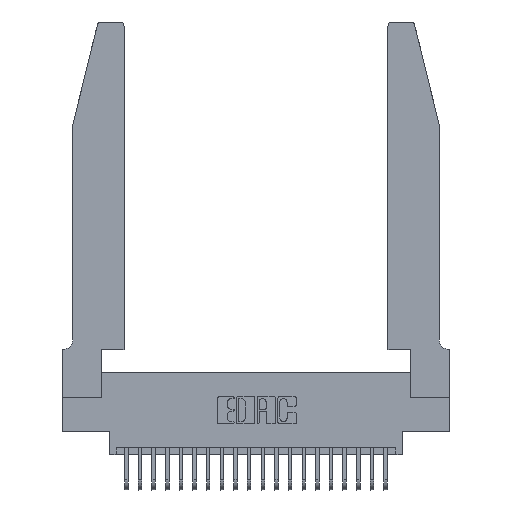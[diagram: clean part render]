
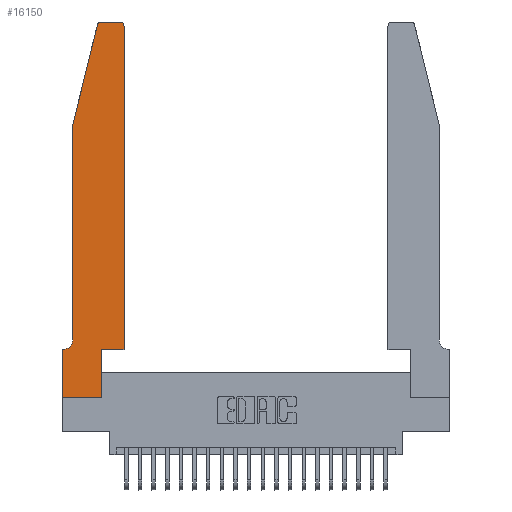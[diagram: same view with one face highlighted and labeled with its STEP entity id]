
A CAD part, top view. The second image highlights one B-rep face of the part: STEP entity #16150.
In plain terms, the highlighted planar face has unit normal (0, 0, 1).
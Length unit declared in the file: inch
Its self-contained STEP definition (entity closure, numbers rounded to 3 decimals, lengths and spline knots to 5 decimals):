
#23 = CARTESIAN_POINT ( 'NONE',  ( 0.25487, 2.72718, 0.37 ) ) ;
#61 = VERTEX_POINT ( 'NONE', #21375 ) ;
#76 = EDGE_CURVE ( 'NONE', #13377, #61, #11208, .T. ) ;
#625 = EDGE_LOOP ( 'NONE', ( #3779, #20470, #11960, #14670, #16155, #15663, #4554, #1819, #11596, #8665, #4752, #5791 ) ) ;
#868 = DIRECTION ( 'NONE',  ( -0.239, -0.971, 0. ) ) ;
#911 = EDGE_CURVE ( 'NONE', #7710, #11532, #14795, .T. ) ;
#967 = LINE ( 'NONE', #7769, #9959 ) ;
#1411 = DIRECTION ( 'NONE',  ( -1., 0., 0. ) ) ;
#1785 = VERTEX_POINT ( 'NONE', #6519 ) ;
#1819 = ORIENTED_EDGE ( 'NONE', *, *, #5611, .T. ) ;
#1923 = CARTESIAN_POINT ( 'NONE',  ( 0.2865, 0.35, 0.37 ) ) ;
#2019 = DIRECTION ( 'NONE',  ( 0., 0., 1. ) ) ;
#3181 = CARTESIAN_POINT ( 'NONE',  ( 0.2865, 0., 0.37 ) ) ;
#3467 = VECTOR ( 'NONE', #868, 39.37008 ) ;
#3557 = LINE ( 'NONE', #11587, #8333 ) ;
#3666 = DIRECTION ( 'NONE',  ( 0., 1., 0. ) ) ;
#3731 = CARTESIAN_POINT ( 'NONE',  ( 0., 0.35, 0.37 ) ) ;
#3779 = ORIENTED_EDGE ( 'NONE', *, *, #5363, .T. ) ;
#3974 = VERTEX_POINT ( 'NONE', #16724 ) ;
#4528 = EDGE_CURVE ( 'NONE', #19229, #3974, #967, .T. ) ;
#4554 = ORIENTED_EDGE ( 'NONE', *, *, #14493, .T. ) ;
#4644 = EDGE_CURVE ( 'NONE', #18680, #19229, #3557, .T. ) ;
#4752 = ORIENTED_EDGE ( 'NONE', *, *, #4528, .T. ) ;
#4996 = EDGE_CURVE ( 'NONE', #8780, #18680, #18169, .T. ) ;
#5137 = VERTEX_POINT ( 'NONE', #11493 ) ;
#5363 = EDGE_CURVE ( 'NONE', #1785, #21702, #6318, .T. ) ;
#5474 = CARTESIAN_POINT ( 'NONE',  ( 0.4505, 0.35, 0.37 ) ) ;
#5552 = DIRECTION ( 'NONE',  ( 1., 0., 0. ) ) ;
#5611 = EDGE_CURVE ( 'NONE', #5137, #8780, #15953, .T. ) ;
#5791 = ORIENTED_EDGE ( 'NONE', *, *, #6215, .T. ) ;
#6003 = AXIS2_PLACEMENT_3D ( 'NONE', #12682, #2019, #14461 ) ;
#6215 = EDGE_CURVE ( 'NONE', #3974, #1785, #21952, .T. ) ;
#6318 = LINE ( 'NONE', #15631, #11018 ) ;
#6483 = EDGE_CURVE ( 'NONE', #10696, #13377, #19195, .T. ) ;
#6511 = VECTOR ( 'NONE', #15217, 39.37008 ) ;
#6519 = CARTESIAN_POINT ( 'NONE',  ( 0.4205, 2.75, 0.37 ) ) ;
#7412 = DIRECTION ( 'NONE',  ( 1., 0., 0. ) ) ;
#7710 = VERTEX_POINT ( 'NONE', #10465 ) ;
#7769 = CARTESIAN_POINT ( 'NONE',  ( 0.4505, 0.35, 0.37 ) ) ;
#8023 = DIRECTION ( 'NONE',  ( -1., 0., 0. ) ) ;
#8079 = DIRECTION ( 'NONE',  ( 1., 0., 0. ) ) ;
#8243 = CARTESIAN_POINT ( 'NONE',  ( 0., 0.35, 0.37 ) ) ;
#8333 = VECTOR ( 'NONE', #8079, 39.37008 ) ;
#8665 = ORIENTED_EDGE ( 'NONE', *, *, #4644, .T. ) ;
#8780 = VERTEX_POINT ( 'NONE', #3181 ) ;
#8869 = VECTOR ( 'NONE', #3666, 39.37008 ) ;
#8894 = DIRECTION ( 'NONE',  ( 0., 0., 1. ) ) ;
#9206 = CARTESIAN_POINT ( 'NONE',  ( 0., 0., 0.37 ) ) ;
#9245 = DIRECTION ( 'NONE',  ( 0., -1., 0. ) ) ;
#9709 = VECTOR ( 'NONE', #9245, 39.37008 ) ;
#9959 = VECTOR ( 'NONE', #21789, 39.37008 ) ;
#10465 = CARTESIAN_POINT ( 'NONE',  ( 0.0055, 0.35, 0.37 ) ) ;
#10591 = CARTESIAN_POINT ( 'NONE',  ( 0.0055, 0.42, 0.37 ) ) ;
#10614 = EDGE_CURVE ( 'NONE', #21702, #10696, #13562, .T. ) ;
#10696 = VERTEX_POINT ( 'NONE', #23 ) ;
#11018 = VECTOR ( 'NONE', #1411, 39.37008 ) ;
#11208 = LINE ( 'NONE', #15834, #6511 ) ;
#11493 = CARTESIAN_POINT ( 'NONE',  ( 0., 0., 0.37 ) ) ;
#11532 = VERTEX_POINT ( 'NONE', #8243 ) ;
#11587 = CARTESIAN_POINT ( 'NONE',  ( 0.4505, 0.35, 0.37 ) ) ;
#11591 = CARTESIAN_POINT ( 'NONE',  ( 0.0755, 2., 0.37 ) ) ;
#11596 = ORIENTED_EDGE ( 'NONE', *, *, #4996, .T. ) ;
#11960 = ORIENTED_EDGE ( 'NONE', *, *, #6483, .T. ) ;
#12363 = DIRECTION ( 'NONE',  ( -1., 0., 0. ) ) ;
#12557 = PLANE ( 'NONE',  #21148 ) ;
#12671 = CARTESIAN_POINT ( 'NONE',  ( 0., 0., 0.37 ) ) ;
#12682 = CARTESIAN_POINT ( 'NONE',  ( 0.4205, 2.72, 0.37 ) ) ;
#13347 = CARTESIAN_POINT ( 'NONE',  ( 0.0755, 0.35, 0.37 ) ) ;
#13377 = VERTEX_POINT ( 'NONE', #16473 ) ;
#13562 = CIRCLE ( 'NONE', #15206, 0.03 ) ;
#14337 = EDGE_CURVE ( 'NONE', #61, #7710, #22563, .T. ) ;
#14461 = DIRECTION ( 'NONE',  ( 1., 0., 0. ) ) ;
#14493 = EDGE_CURVE ( 'NONE', #11532, #5137, #19025, .T. ) ;
#14670 = ORIENTED_EDGE ( 'NONE', *, *, #76, .T. ) ;
#14795 = LINE ( 'NONE', #13347, #18893 ) ;
#15108 = AXIS2_PLACEMENT_3D ( 'NONE', #10591, #22869, #12363 ) ;
#15206 = AXIS2_PLACEMENT_3D ( 'NONE', #19372, #8894, #21140 ) ;
#15217 = DIRECTION ( 'NONE',  ( 0., -1., 0. ) ) ;
#15631 = CARTESIAN_POINT ( 'NONE',  ( 0.2605, 2.75, 0.37 ) ) ;
#15663 = ORIENTED_EDGE ( 'NONE', *, *, #911, .T. ) ;
#15834 = CARTESIAN_POINT ( 'NONE',  ( 0.0755, 2., 0.37 ) ) ;
#15953 = LINE ( 'NONE', #9206, #20076 ) ;
#16089 = DIRECTION ( 'NONE',  ( 0., 0., 1. ) ) ;
#16150 = ADVANCED_FACE ( 'NONE', ( #20584 ), #12557, .T. ) ;
#16155 = ORIENTED_EDGE ( 'NONE', *, *, #14337, .T. ) ;
#16473 = CARTESIAN_POINT ( 'NONE',  ( 0.0755, 2., 0.37 ) ) ;
#16724 = CARTESIAN_POINT ( 'NONE',  ( 0.4505, 2.72, 0.37 ) ) ;
#18169 = LINE ( 'NONE', #21239, #8869 ) ;
#18680 = VERTEX_POINT ( 'NONE', #1923 ) ;
#18893 = VECTOR ( 'NONE', #8023, 39.37008 ) ;
#19025 = LINE ( 'NONE', #12671, #9709 ) ;
#19195 = LINE ( 'NONE', #11591, #3467 ) ;
#19229 = VERTEX_POINT ( 'NONE', #5474 ) ;
#19372 = CARTESIAN_POINT ( 'NONE',  ( 0.284, 2.72, 0.37 ) ) ;
#20076 = VECTOR ( 'NONE', #7412, 39.37008 ) ;
#20470 = ORIENTED_EDGE ( 'NONE', *, *, #10614, .T. ) ;
#20584 = FACE_OUTER_BOUND ( 'NONE', #625, .T. ) ;
#20707 = CARTESIAN_POINT ( 'NONE',  ( 0.284, 2.75, 0.37 ) ) ;
#21140 = DIRECTION ( 'NONE',  ( 1., 0., 0. ) ) ;
#21148 = AXIS2_PLACEMENT_3D ( 'NONE', #3731, #16089, #5552 ) ;
#21239 = CARTESIAN_POINT ( 'NONE',  ( 0.2865, 0.35, 0.37 ) ) ;
#21375 = CARTESIAN_POINT ( 'NONE',  ( 0.0755, 0.42, 0.37 ) ) ;
#21702 = VERTEX_POINT ( 'NONE', #20707 ) ;
#21789 = DIRECTION ( 'NONE',  ( 0., 1., 0. ) ) ;
#21952 = CIRCLE ( 'NONE', #6003, 0.03 ) ;
#22563 = CIRCLE ( 'NONE', #15108, 0.07 ) ;
#22869 = DIRECTION ( 'NONE',  ( 0., 0., -1. ) ) ;
